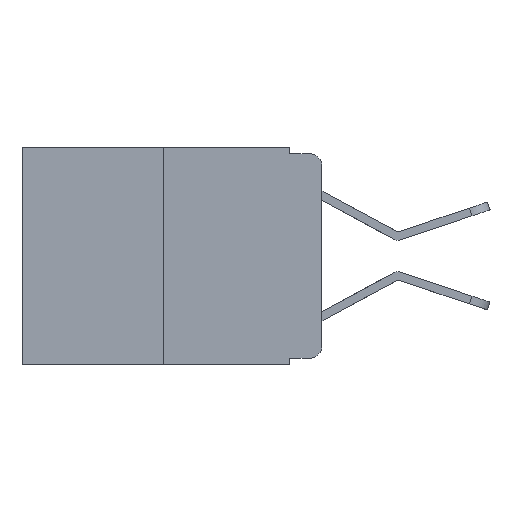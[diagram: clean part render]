
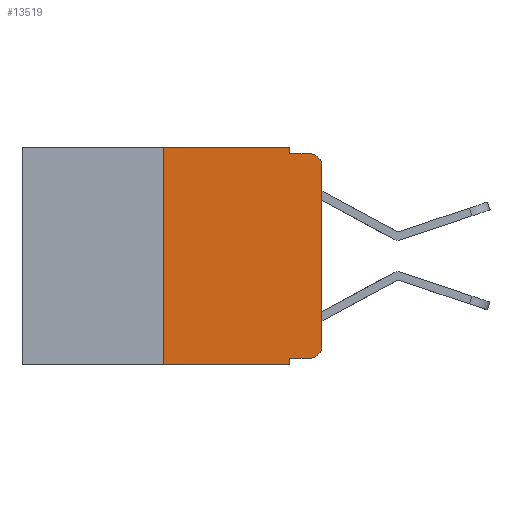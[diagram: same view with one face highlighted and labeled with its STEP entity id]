
A CAD part, left-side view. The second image highlights one B-rep face of the part: STEP entity #13519.
In plain terms, the highlighted planar face has unit normal (-1, 0, 0).
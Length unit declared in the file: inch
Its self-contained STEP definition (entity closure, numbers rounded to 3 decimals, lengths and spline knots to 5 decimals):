
#141 = DIRECTION ( 'NONE',  ( 0., 0., -1. ) ) ;
#166 = CIRCLE ( 'NONE', #15295, 0.02 ) ;
#220 = CARTESIAN_POINT ( 'NONE',  ( 0., 0.25, 0. ) ) ;
#231 = LINE ( 'NONE', #220, #19964 ) ;
#332 = CARTESIAN_POINT ( 'NONE',  ( 0., 0.25, -0.343 ) ) ;
#385 = LINE ( 'NONE', #11320, #3883 ) ;
#939 = LINE ( 'NONE', #1678, #16936 ) ;
#1678 = CARTESIAN_POINT ( 'NONE',  ( 0., 0.051, 0. ) ) ;
#1746 = DIRECTION ( 'NONE',  ( 0., -1., 0. ) ) ;
#2033 = DIRECTION ( 'NONE',  ( 0., 0., -1. ) ) ;
#2853 = DIRECTION ( 'NONE',  ( 0., -1., 0. ) ) ;
#2872 = VERTEX_POINT ( 'NONE', #7587 ) ;
#3030 = CARTESIAN_POINT ( 'NONE',  ( 0., 0.02, -0.313 ) ) ;
#3045 = CIRCLE ( 'NONE', #7204, 0.02 ) ;
#3097 = CARTESIAN_POINT ( 'NONE',  ( 0., 0.051, -0.01 ) ) ;
#3360 = PLANE ( 'NONE',  #4142 ) ;
#3374 = DIRECTION ( 'NONE',  ( 0., 0., 1. ) ) ;
#3883 = VECTOR ( 'NONE', #1746, 39.37008 ) ;
#4142 = AXIS2_PLACEMENT_3D ( 'NONE', #12799, #4621, #17594 ) ;
#4168 = VERTEX_POINT ( 'NONE', #10825 ) ;
#4393 = CARTESIAN_POINT ( 'NONE',  ( 0., 0.02, -0.03 ) ) ;
#4621 = DIRECTION ( 'NONE',  ( 1., 0., 0. ) ) ;
#4996 = CARTESIAN_POINT ( 'NONE',  ( 0., 0.02, -0.01 ) ) ;
#5021 = VERTEX_POINT ( 'NONE', #11869 ) ;
#5223 = EDGE_CURVE ( 'NONE', #2872, #18477, #166, .T. ) ;
#5513 = ORIENTED_EDGE ( 'NONE', *, *, #17114, .T. ) ;
#5546 = LINE ( 'NONE', #14240, #14800 ) ;
#6357 = ORIENTED_EDGE ( 'NONE', *, *, #5223, .T. ) ;
#6428 = CARTESIAN_POINT ( 'NONE',  ( 0., 0., -0.03 ) ) ;
#6654 = CARTESIAN_POINT ( 'NONE',  ( 0., 0.051, 0. ) ) ;
#6733 = FACE_OUTER_BOUND ( 'NONE', #20098, .T. ) ;
#7204 = AXIS2_PLACEMENT_3D ( 'NONE', #4393, #7565, #15578 ) ;
#7518 = VERTEX_POINT ( 'NONE', #13517 ) ;
#7565 = DIRECTION ( 'NONE',  ( -1., 0., 0. ) ) ;
#7587 = CARTESIAN_POINT ( 'NONE',  ( 0., 0.02, -0.333 ) ) ;
#7733 = DIRECTION ( 'NONE',  ( 0., -1., 0. ) ) ;
#7773 = VERTEX_POINT ( 'NONE', #332 ) ;
#7775 = EDGE_CURVE ( 'NONE', #20108, #5021, #9122, .T. ) ;
#8443 = ORIENTED_EDGE ( 'NONE', *, *, #10476, .T. ) ;
#9122 = LINE ( 'NONE', #6654, #18555 ) ;
#9275 = DIRECTION ( 'NONE',  ( -1., 0., 0. ) ) ;
#9774 = VECTOR ( 'NONE', #10579, 39.37008 ) ;
#10109 = VERTEX_POINT ( 'NONE', #6428 ) ;
#10476 = EDGE_CURVE ( 'NONE', #10109, #11916, #3045, .T. ) ;
#10579 = DIRECTION ( 'NONE',  ( 0., -1., 0. ) ) ;
#10600 = CARTESIAN_POINT ( 'NONE',  ( 0., 0., -0.313 ) ) ;
#10825 = CARTESIAN_POINT ( 'NONE',  ( 0., 0.25, 0. ) ) ;
#10993 = EDGE_CURVE ( 'NONE', #18477, #10109, #5546, .T. ) ;
#11320 = CARTESIAN_POINT ( 'NONE',  ( 0., 0.473, 0. ) ) ;
#11668 = LINE ( 'NONE', #12427, #18891 ) ;
#11812 = EDGE_CURVE ( 'NONE', #19409, #11916, #15007, .T. ) ;
#11869 = CARTESIAN_POINT ( 'NONE',  ( 0., 0.051, -0.343 ) ) ;
#11901 = EDGE_CURVE ( 'NONE', #7773, #4168, #231, .T. ) ;
#11916 = VERTEX_POINT ( 'NONE', #4996 ) ;
#11971 = ORIENTED_EDGE ( 'NONE', *, *, #7775, .F. ) ;
#12084 = CARTESIAN_POINT ( 'NONE',  ( 0., 0.051, -0.333 ) ) ;
#12427 = CARTESIAN_POINT ( 'NONE',  ( 0., 0.051, -0.333 ) ) ;
#12799 = CARTESIAN_POINT ( 'NONE',  ( 0., 0.473, 0. ) ) ;
#12830 = ORIENTED_EDGE ( 'NONE', *, *, #11901, .F. ) ;
#13022 = LINE ( 'NONE', #16744, #9774 ) ;
#13517 = CARTESIAN_POINT ( 'NONE',  ( 0., 0.051, 0. ) ) ;
#13519 = ADVANCED_FACE ( 'NONE', ( #6733 ), #3360, .F. ) ;
#14150 = ORIENTED_EDGE ( 'NONE', *, *, #10993, .T. ) ;
#14217 = DIRECTION ( 'NONE',  ( 0., 0., -1. ) ) ;
#14240 = CARTESIAN_POINT ( 'NONE',  ( 0., 0., 0. ) ) ;
#14800 = VECTOR ( 'NONE', #15704, 39.37008 ) ;
#14929 = EDGE_CURVE ( 'NONE', #4168, #7518, #385, .T. ) ;
#15007 = LINE ( 'NONE', #3097, #19481 ) ;
#15295 = AXIS2_PLACEMENT_3D ( 'NONE', #3030, #9275, #14217 ) ;
#15578 = DIRECTION ( 'NONE',  ( 0., 0., -1. ) ) ;
#15704 = DIRECTION ( 'NONE',  ( 0., 0., 1. ) ) ;
#15940 = ORIENTED_EDGE ( 'NONE', *, *, #11812, .F. ) ;
#15943 = ORIENTED_EDGE ( 'NONE', *, *, #19857, .F. ) ;
#16744 = CARTESIAN_POINT ( 'NONE',  ( 0., 0.473, -0.343 ) ) ;
#16936 = VECTOR ( 'NONE', #141, 39.37008 ) ;
#17114 = EDGE_CURVE ( 'NONE', #7773, #5021, #13022, .T. ) ;
#17594 = DIRECTION ( 'NONE',  ( 0., 0., -1. ) ) ;
#18349 = ORIENTED_EDGE ( 'NONE', *, *, #19480, .T. ) ;
#18477 = VERTEX_POINT ( 'NONE', #10600 ) ;
#18555 = VECTOR ( 'NONE', #2033, 39.37008 ) ;
#18891 = VECTOR ( 'NONE', #2853, 39.37008 ) ;
#19409 = VERTEX_POINT ( 'NONE', #19693 ) ;
#19480 = EDGE_CURVE ( 'NONE', #20108, #2872, #11668, .T. ) ;
#19481 = VECTOR ( 'NONE', #7733, 39.37008 ) ;
#19693 = CARTESIAN_POINT ( 'NONE',  ( 0., 0.051, -0.01 ) ) ;
#19748 = ORIENTED_EDGE ( 'NONE', *, *, #14929, .F. ) ;
#19857 = EDGE_CURVE ( 'NONE', #7518, #19409, #939, .T. ) ;
#19964 = VECTOR ( 'NONE', #3374, 39.37008 ) ;
#20098 = EDGE_LOOP ( 'NONE', ( #14150, #8443, #15940, #15943, #19748, #12830, #5513, #11971, #18349, #6357 ) ) ;
#20108 = VERTEX_POINT ( 'NONE', #12084 ) ;
